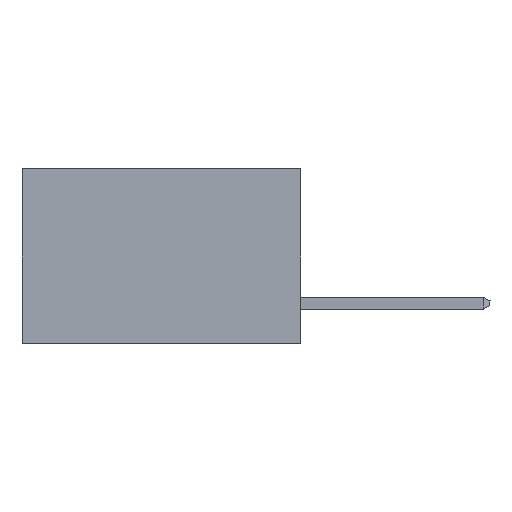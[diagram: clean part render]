
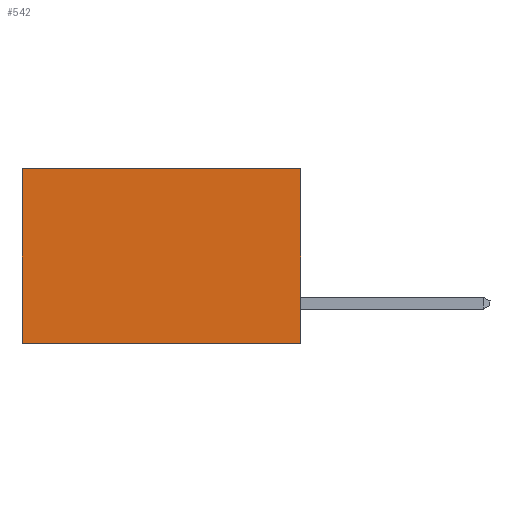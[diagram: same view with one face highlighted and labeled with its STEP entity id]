
A CAD part, left-side view. The second image highlights one B-rep face of the part: STEP entity #542.
In plain terms, the highlighted planar face has unit normal (-1, 0, 0).
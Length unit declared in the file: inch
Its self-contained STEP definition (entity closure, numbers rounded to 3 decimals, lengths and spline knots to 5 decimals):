
#79 = DIRECTION ( 'NONE',  ( 0., 0., -1. ) ) ;
#542 = ADVANCED_FACE ( 'NONE', ( #13465 ), #13771, .F. ) ;
#958 = DIRECTION ( 'NONE',  ( 0., 0., -1. ) ) ;
#1448 = CARTESIAN_POINT ( 'NONE',  ( 0.277, 0.59, -0.37 ) ) ;
#2608 = LINE ( 'NONE', #9968, #8350 ) ;
#3115 = LINE ( 'NONE', #10541, #12115 ) ;
#3310 = EDGE_CURVE ( 'NONE', #9319, #6024, #5961, .T. ) ;
#4044 = CARTESIAN_POINT ( 'NONE',  ( 0.277, 0.59, 0. ) ) ;
#4442 = CARTESIAN_POINT ( 'NONE',  ( 0.277, 0., -0.37 ) ) ;
#4659 = EDGE_CURVE ( 'NONE', #8080, #6024, #3115, .T. ) ;
#4751 = EDGE_CURVE ( 'NONE', #10855, #8080, #5065, .T. ) ;
#5065 = LINE ( 'NONE', #4442, #7776 ) ;
#5618 = VECTOR ( 'NONE', #958, 39.37008 ) ;
#5807 = CARTESIAN_POINT ( 'NONE',  ( 0.277, 0., 0. ) ) ;
#5961 = LINE ( 'NONE', #1448, #5618 ) ;
#6024 = VERTEX_POINT ( 'NONE', #9738 ) ;
#6765 = ORIENTED_EDGE ( 'NONE', *, *, #3310, .T. ) ;
#6928 = EDGE_CURVE ( 'NONE', #10855, #9319, #2608, .T. ) ;
#7776 = VECTOR ( 'NONE', #9697, 39.37008 ) ;
#8080 = VERTEX_POINT ( 'NONE', #13024 ) ;
#8350 = VECTOR ( 'NONE', #10073, 39.37008 ) ;
#8485 = EDGE_LOOP ( 'NONE', ( #6765, #9984, #9301, #8924 ) ) ;
#8749 = DIRECTION ( 'NONE',  ( 0., 1., 0. ) ) ;
#8924 = ORIENTED_EDGE ( 'NONE', *, *, #6928, .T. ) ;
#9301 = ORIENTED_EDGE ( 'NONE', *, *, #4751, .F. ) ;
#9319 = VERTEX_POINT ( 'NONE', #4044 ) ;
#9697 = DIRECTION ( 'NONE',  ( 0., 0., -1. ) ) ;
#9738 = CARTESIAN_POINT ( 'NONE',  ( 0.277, 0.59, -0.37 ) ) ;
#9968 = CARTESIAN_POINT ( 'NONE',  ( 0.277, 0., 0. ) ) ;
#9984 = ORIENTED_EDGE ( 'NONE', *, *, #4659, .F. ) ;
#10073 = DIRECTION ( 'NONE',  ( 0., 1., 0. ) ) ;
#10541 = CARTESIAN_POINT ( 'NONE',  ( 0.277, 0., -0.37 ) ) ;
#10654 = AXIS2_PLACEMENT_3D ( 'NONE', #12934, #11723, #79 ) ;
#10855 = VERTEX_POINT ( 'NONE', #5807 ) ;
#11723 = DIRECTION ( 'NONE',  ( 1., 0., 0. ) ) ;
#12115 = VECTOR ( 'NONE', #8749, 39.37008 ) ;
#12934 = CARTESIAN_POINT ( 'NONE',  ( 0.277, 0., -0.37 ) ) ;
#13024 = CARTESIAN_POINT ( 'NONE',  ( 0.277, 0., -0.37 ) ) ;
#13465 = FACE_OUTER_BOUND ( 'NONE', #8485, .T. ) ;
#13771 = PLANE ( 'NONE',  #10654 ) ;
